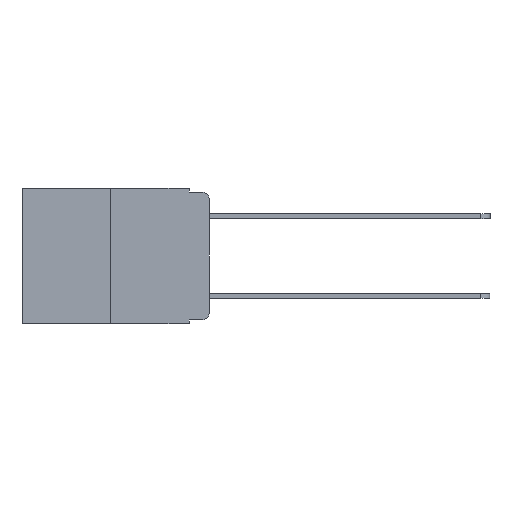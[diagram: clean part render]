
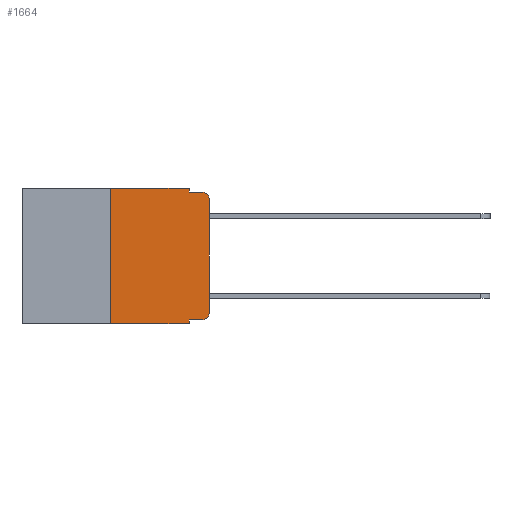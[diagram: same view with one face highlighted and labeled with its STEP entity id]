
A CAD part, left-side view. The second image highlights one B-rep face of the part: STEP entity #1664.
In plain terms, the highlighted planar face has unit normal (-1, 0, 0).
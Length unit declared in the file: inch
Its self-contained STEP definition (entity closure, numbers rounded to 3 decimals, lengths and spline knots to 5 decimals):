
#101 = CARTESIAN_POINT ( 'NONE',  ( 0., 0.473, -0.343 ) ) ;
#163 = VECTOR ( 'NONE', #6413, 39.37008 ) ;
#188 = EDGE_CURVE ( 'NONE', #4367, #7756, #3487, .T. ) ;
#239 = ORIENTED_EDGE ( 'NONE', *, *, #188, .T. ) ;
#311 = DIRECTION ( 'NONE',  ( -1., 0., 0. ) ) ;
#312 = EDGE_CURVE ( 'NONE', #6855, #8949, #4281, .T. ) ;
#327 = CARTESIAN_POINT ( 'NONE',  ( 0., 0.02, -0.313 ) ) ;
#333 = ORIENTED_EDGE ( 'NONE', *, *, #6505, .T. ) ;
#647 = CARTESIAN_POINT ( 'NONE',  ( 0., 0.02, -0.333 ) ) ;
#653 = ORIENTED_EDGE ( 'NONE', *, *, #7186, .F. ) ;
#659 = AXIS2_PLACEMENT_3D ( 'NONE', #327, #311, #7298 ) ;
#664 = ORIENTED_EDGE ( 'NONE', *, *, #5102, .F. ) ;
#710 = VECTOR ( 'NONE', #8601, 39.37008 ) ;
#813 = CARTESIAN_POINT ( 'NONE',  ( 0., 0.25, -0.343 ) ) ;
#867 = LINE ( 'NONE', #8454, #8380 ) ;
#985 = DIRECTION ( 'NONE',  ( 0., 0., -1. ) ) ;
#1009 = DIRECTION ( 'NONE',  ( -1., 0., 0. ) ) ;
#1037 = CARTESIAN_POINT ( 'NONE',  ( 0., 0.02, -0.01 ) ) ;
#1076 = EDGE_LOOP ( 'NONE', ( #2854, #239, #9321, #653, #1666, #5109, #7554, #664, #4809, #333 ) ) ;
#1099 = CARTESIAN_POINT ( 'NONE',  ( 0., 0.02, -0.03 ) ) ;
#1591 = VERTEX_POINT ( 'NONE', #6261 ) ;
#1664 = ADVANCED_FACE ( 'NONE', ( #7040 ), #4470, .F. ) ;
#1666 = ORIENTED_EDGE ( 'NONE', *, *, #312, .F. ) ;
#1799 = EDGE_CURVE ( 'NONE', #7593, #7756, #4015, .T. ) ;
#1843 = LINE ( 'NONE', #101, #2096 ) ;
#1859 = DIRECTION ( 'NONE',  ( 0., 0., 1. ) ) ;
#2075 = DIRECTION ( 'NONE',  ( 0., 0., -1. ) ) ;
#2096 = VECTOR ( 'NONE', #8175, 39.37008 ) ;
#2449 = VERTEX_POINT ( 'NONE', #647 ) ;
#2478 = VECTOR ( 'NONE', #8212, 39.37008 ) ;
#2651 = EDGE_CURVE ( 'NONE', #3590, #6855, #4606, .T. ) ;
#2854 = ORIENTED_EDGE ( 'NONE', *, *, #7809, .T. ) ;
#3046 = CARTESIAN_POINT ( 'NONE',  ( 0., 0.051, 0. ) ) ;
#3294 = CARTESIAN_POINT ( 'NONE',  ( 0., 0.051, 0. ) ) ;
#3359 = CARTESIAN_POINT ( 'NONE',  ( 0., 0.473, 0. ) ) ;
#3487 = CIRCLE ( 'NONE', #5523, 0.02 ) ;
#3590 = VERTEX_POINT ( 'NONE', #813 ) ;
#4015 = LINE ( 'NONE', #4511, #7567 ) ;
#4281 = LINE ( 'NONE', #8552, #710 ) ;
#4318 = DIRECTION ( 'NONE',  ( 0., -1., 0. ) ) ;
#4367 = VERTEX_POINT ( 'NONE', #8932 ) ;
#4470 = PLANE ( 'NONE',  #7950 ) ;
#4478 = DIRECTION ( 'NONE',  ( 1., 0., 0. ) ) ;
#4511 = CARTESIAN_POINT ( 'NONE',  ( 0., 0.051, -0.01 ) ) ;
#4592 = VERTEX_POINT ( 'NONE', #8337 ) ;
#4606 = LINE ( 'NONE', #7532, #8097 ) ;
#4640 = CARTESIAN_POINT ( 'NONE',  ( 0., 0.051, -0.343 ) ) ;
#4809 = ORIENTED_EDGE ( 'NONE', *, *, #7929, .T. ) ;
#4915 = CARTESIAN_POINT ( 'NONE',  ( 0., 0.051, 0. ) ) ;
#5102 = EDGE_CURVE ( 'NONE', #1591, #8259, #6403, .T. ) ;
#5109 = ORIENTED_EDGE ( 'NONE', *, *, #2651, .F. ) ;
#5523 = AXIS2_PLACEMENT_3D ( 'NONE', #1099, #1009, #985 ) ;
#5686 = DIRECTION ( 'NONE',  ( 0., -1., 0. ) ) ;
#5743 = CARTESIAN_POINT ( 'NONE',  ( 0., 0.25, 0. ) ) ;
#5995 = LINE ( 'NONE', #9015, #7852 ) ;
#6120 = LINE ( 'NONE', #4915, #2478 ) ;
#6261 = CARTESIAN_POINT ( 'NONE',  ( 0., 0.051, -0.333 ) ) ;
#6403 = LINE ( 'NONE', #3046, #163 ) ;
#6413 = DIRECTION ( 'NONE',  ( 0., 0., -1. ) ) ;
#6505 = EDGE_CURVE ( 'NONE', #2449, #4592, #6897, .T. ) ;
#6832 = DIRECTION ( 'NONE',  ( 0., 0., 1. ) ) ;
#6855 = VERTEX_POINT ( 'NONE', #5743 ) ;
#6897 = CIRCLE ( 'NONE', #659, 0.02 ) ;
#7040 = FACE_OUTER_BOUND ( 'NONE', #1076, .T. ) ;
#7186 = EDGE_CURVE ( 'NONE', #8949, #7593, #6120, .T. ) ;
#7271 = CARTESIAN_POINT ( 'NONE',  ( 0., 0.051, -0.01 ) ) ;
#7298 = DIRECTION ( 'NONE',  ( 0., 0., -1. ) ) ;
#7532 = CARTESIAN_POINT ( 'NONE',  ( 0., 0.25, 0. ) ) ;
#7554 = ORIENTED_EDGE ( 'NONE', *, *, #8311, .T. ) ;
#7567 = VECTOR ( 'NONE', #4318, 39.37008 ) ;
#7593 = VERTEX_POINT ( 'NONE', #7271 ) ;
#7756 = VERTEX_POINT ( 'NONE', #1037 ) ;
#7809 = EDGE_CURVE ( 'NONE', #4592, #4367, #5995, .T. ) ;
#7852 = VECTOR ( 'NONE', #1859, 39.37008 ) ;
#7929 = EDGE_CURVE ( 'NONE', #1591, #2449, #867, .T. ) ;
#7950 = AXIS2_PLACEMENT_3D ( 'NONE', #3359, #4478, #2075 ) ;
#8097 = VECTOR ( 'NONE', #6832, 39.37008 ) ;
#8175 = DIRECTION ( 'NONE',  ( 0., -1., 0. ) ) ;
#8212 = DIRECTION ( 'NONE',  ( 0., 0., -1. ) ) ;
#8259 = VERTEX_POINT ( 'NONE', #4640 ) ;
#8311 = EDGE_CURVE ( 'NONE', #3590, #8259, #1843, .T. ) ;
#8337 = CARTESIAN_POINT ( 'NONE',  ( 0., 0., -0.313 ) ) ;
#8380 = VECTOR ( 'NONE', #5686, 39.37008 ) ;
#8454 = CARTESIAN_POINT ( 'NONE',  ( 0., 0.051, -0.333 ) ) ;
#8552 = CARTESIAN_POINT ( 'NONE',  ( 0., 0.473, 0. ) ) ;
#8601 = DIRECTION ( 'NONE',  ( 0., -1., 0. ) ) ;
#8932 = CARTESIAN_POINT ( 'NONE',  ( 0., 0., -0.03 ) ) ;
#8949 = VERTEX_POINT ( 'NONE', #3294 ) ;
#9015 = CARTESIAN_POINT ( 'NONE',  ( 0., 0., 0. ) ) ;
#9321 = ORIENTED_EDGE ( 'NONE', *, *, #1799, .F. ) ;
